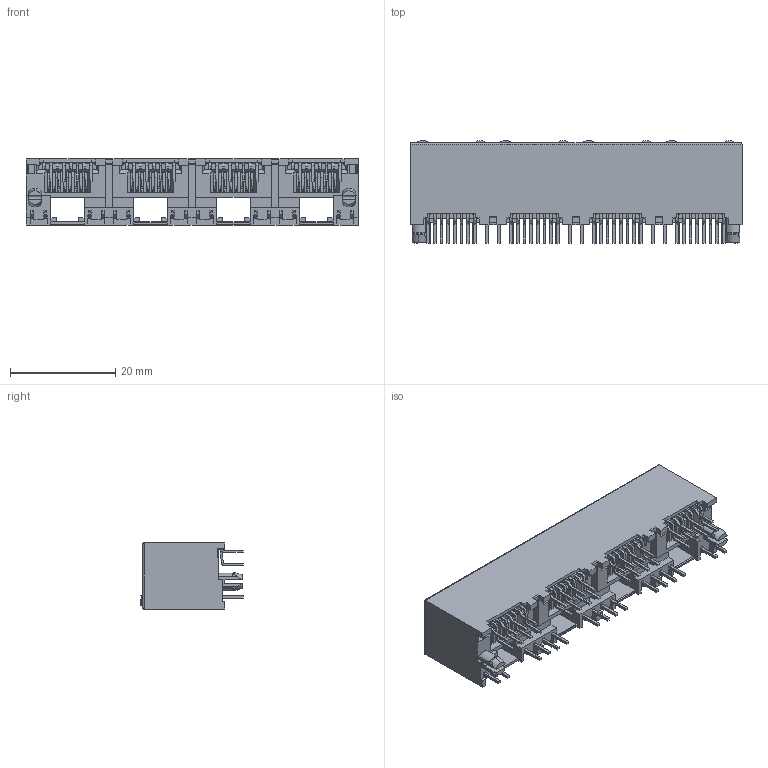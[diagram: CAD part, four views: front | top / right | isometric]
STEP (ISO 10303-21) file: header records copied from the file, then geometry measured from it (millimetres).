
FILE_DESCRIPTION (( 'STEP AP203' ), '1' );
FILE_NAME ('J2W048821N51031.STEP', '2020-10-05T20:30:33', ( '' ), ( '' ), 'SwSTEP 2.0', 'SolidWorks 2020', '' );
FILE_SCHEMA (( 'CONFIG_CONTROL_DESIGN' ));
Length unit declared in the file: millimetre
Products named in the file (6): 2W LED RH_1-Yellow; 2W LED LH_5-Green-Yellow; 2W Contacts; 2W Contact Lock; J2W048821N51031; 2W Insulator
Assembly tree (17 placements, depth 2):
  J2W048821N51031
    2W Insulator
    2W Contacts  x4
    2W Contact Lock  x4
    2W LED LH_5-Green-Yellow  x4
    2W LED RH_1-Yellow  x4
Bounding box: 63 x 19.5 x 12.55 mm (x, y, z)
Volume: 5334.9 mm3; surface area: 13143.9 mm2
Topology: 45 solids, 45 shells, 3139 faces, 9170 edges, 6009 vertices
Faces by surface type: plane 2600, cylinder 481, bspline 47, cone 11
Entity records: 70315 total; most frequent: CARTESIAN_POINT 23915, ORIENTED_EDGE 11452, DIRECTION 6516, EDGE_CURVE 5726, VERTEX_POINT 3735, B_SPLINE_CURVE_WITH_KNOTS 3172, VECTOR 2352, LINE 2352
